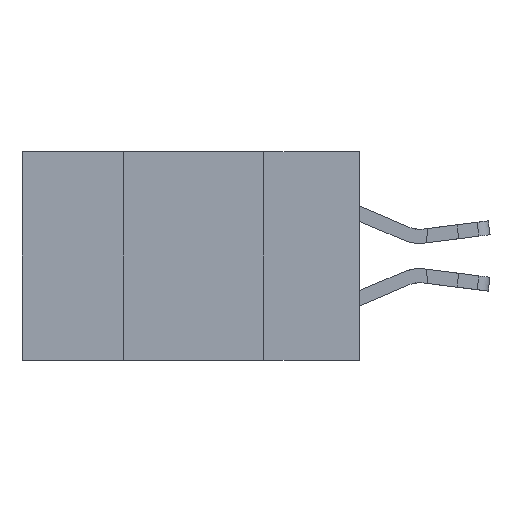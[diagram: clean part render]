
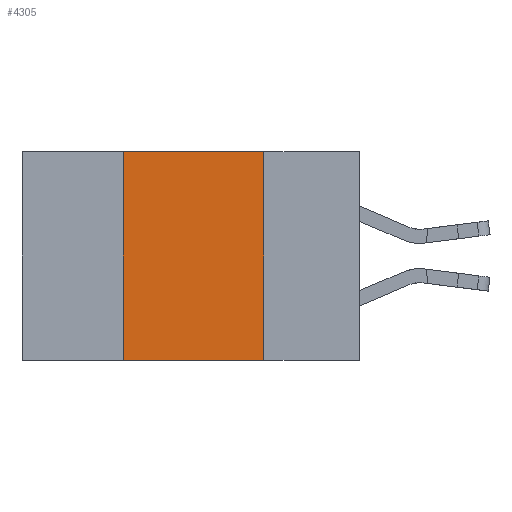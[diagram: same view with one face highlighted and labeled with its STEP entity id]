
A CAD part, left-side view. The second image highlights one B-rep face of the part: STEP entity #4305.
In plain terms, the highlighted planar face has unit normal (-1, 0, 0).
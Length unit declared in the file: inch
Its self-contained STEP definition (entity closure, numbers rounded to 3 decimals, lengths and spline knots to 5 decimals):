
#820 = LINE ( 'NONE', #7776, #10223 ) ;
#831 = VERTEX_POINT ( 'NONE', #3401 ) ;
#909 = CARTESIAN_POINT ( 'NONE',  ( 0., 0.42, -0.37 ) ) ;
#999 = ORIENTED_EDGE ( 'NONE', *, *, #11717, .F. ) ;
#1035 = ORIENTED_EDGE ( 'NONE', *, *, #15019, .F. ) ;
#1153 = ORIENTED_EDGE ( 'NONE', *, *, #10985, .F. ) ;
#1331 = ORIENTED_EDGE ( 'NONE', *, *, #10242, .T. ) ;
#1732 = DIRECTION ( 'NONE',  ( 0., -1., 0. ) ) ;
#2706 = AXIS2_PLACEMENT_3D ( 'NONE', #13121, #13090, #13087 ) ;
#2997 = CARTESIAN_POINT ( 'NONE',  ( 0., 0.42, 0. ) ) ;
#3401 = CARTESIAN_POINT ( 'NONE',  ( 0., 0.17, -0.37 ) ) ;
#4305 = ADVANCED_FACE ( 'NONE', ( #9417 ), #13135, .F. ) ;
#4944 = DIRECTION ( 'NONE',  ( 0., 0., 1. ) ) ;
#5790 = CARTESIAN_POINT ( 'NONE',  ( 0., 0.17, 0. ) ) ;
#6690 = VECTOR ( 'NONE', #1732, 39.37008 ) ;
#7151 = EDGE_LOOP ( 'NONE', ( #999, #1035, #1153, #1331 ) ) ;
#7741 = LINE ( 'NONE', #11452, #10469 ) ;
#7776 = CARTESIAN_POINT ( 'NONE',  ( 0., 0.17, 0. ) ) ;
#7870 = LINE ( 'NONE', #8220, #6690 ) ;
#8220 = CARTESIAN_POINT ( 'NONE',  ( 0., 0.6, -0.37 ) ) ;
#8813 = VECTOR ( 'NONE', #4944, 39.37008 ) ;
#9417 = FACE_OUTER_BOUND ( 'NONE', #7151, .T. ) ;
#10223 = VECTOR ( 'NONE', #12302, 39.37008 ) ;
#10242 = EDGE_CURVE ( 'NONE', #15513, #831, #7870, .T. ) ;
#10390 = DIRECTION ( 'NONE',  ( 0., -1., 0. ) ) ;
#10469 = VECTOR ( 'NONE', #10390, 39.37008 ) ;
#10975 = CARTESIAN_POINT ( 'NONE',  ( 0., 0.42, 0. ) ) ;
#10985 = EDGE_CURVE ( 'NONE', #15513, #12643, #11795, .T. ) ;
#11452 = CARTESIAN_POINT ( 'NONE',  ( 0., 0.6, 0. ) ) ;
#11717 = EDGE_CURVE ( 'NONE', #12665, #831, #820, .T. ) ;
#11795 = LINE ( 'NONE', #10975, #8813 ) ;
#12302 = DIRECTION ( 'NONE',  ( 0., 0., -1. ) ) ;
#12643 = VERTEX_POINT ( 'NONE', #2997 ) ;
#12665 = VERTEX_POINT ( 'NONE', #5790 ) ;
#13087 = DIRECTION ( 'NONE',  ( 0., 0., -1. ) ) ;
#13090 = DIRECTION ( 'NONE',  ( 1., 0., 0. ) ) ;
#13121 = CARTESIAN_POINT ( 'NONE',  ( 0., 0.6, 0. ) ) ;
#13135 = PLANE ( 'NONE',  #2706 ) ;
#15019 = EDGE_CURVE ( 'NONE', #12643, #12665, #7741, .T. ) ;
#15513 = VERTEX_POINT ( 'NONE', #909 ) ;
